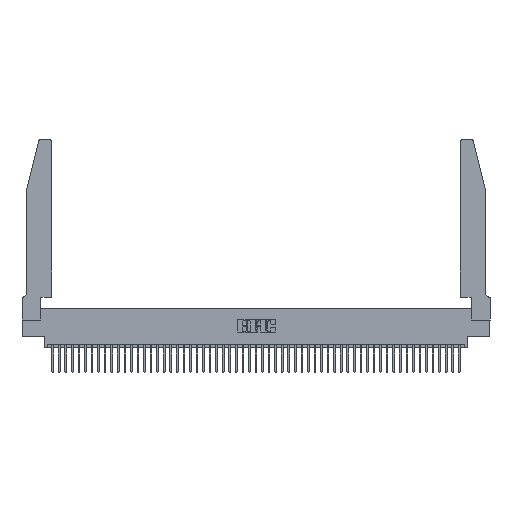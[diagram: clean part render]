
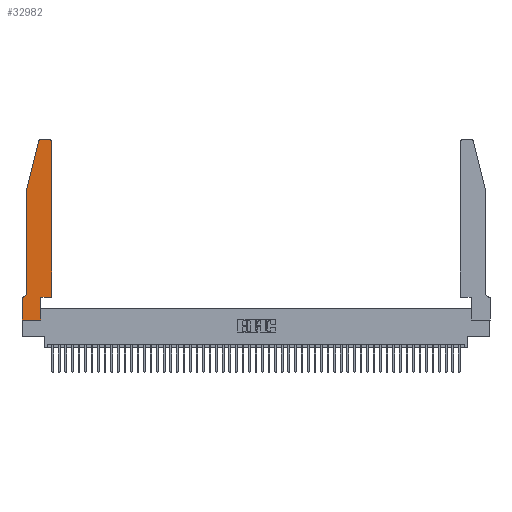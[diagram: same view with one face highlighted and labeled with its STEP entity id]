
A CAD part, top view. The second image highlights one B-rep face of the part: STEP entity #32982.
In plain terms, the highlighted planar face has unit normal (0, 0, 1).
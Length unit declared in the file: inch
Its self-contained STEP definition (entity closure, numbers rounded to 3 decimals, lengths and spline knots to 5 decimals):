
#950 = VERTEX_POINT ( 'NONE', #9124 ) ;
#957 = AXIS2_PLACEMENT_3D ( 'NONE', #36689, #12206, #44151 ) ;
#1061 = CARTESIAN_POINT ( 'NONE',  ( 0.0755, 2., 0.37 ) ) ;
#2277 = LINE ( 'NONE', #39306, #4116 ) ;
#3837 = AXIS2_PLACEMENT_3D ( 'NONE', #20028, #23515, #51494 ) ;
#4067 = ORIENTED_EDGE ( 'NONE', *, *, #48064, .T. ) ;
#4116 = VECTOR ( 'NONE', #31664, 39.37008 ) ;
#4285 = DIRECTION ( 'NONE',  ( 0., 1., 0. ) ) ;
#4808 = CIRCLE ( 'NONE', #3837, 0.03 ) ;
#4816 = DIRECTION ( 'NONE',  ( -1., 0., 0. ) ) ;
#5601 = VERTEX_POINT ( 'NONE', #50166 ) ;
#6028 = LINE ( 'NONE', #1061, #19692 ) ;
#6052 = LINE ( 'NONE', #10722, #41544 ) ;
#6655 = CARTESIAN_POINT ( 'NONE',  ( 0., 0., 0.37 ) ) ;
#6944 = EDGE_CURVE ( 'NONE', #26549, #43588, #12498, .T. ) ;
#7277 = ORIENTED_EDGE ( 'NONE', *, *, #22401, .T. ) ;
#8229 = VERTEX_POINT ( 'NONE', #43483 ) ;
#8336 = EDGE_CURVE ( 'NONE', #22446, #38537, #2277, .T. ) ;
#9124 = CARTESIAN_POINT ( 'NONE',  ( 0.4505, 0.35, 0.37 ) ) ;
#9871 = EDGE_CURVE ( 'NONE', #44445, #32906, #28897, .T. ) ;
#10722 = CARTESIAN_POINT ( 'NONE',  ( 0.2865, 0.35, 0.37 ) ) ;
#11219 = ORIENTED_EDGE ( 'NONE', *, *, #21768, .T. ) ;
#11962 = ORIENTED_EDGE ( 'NONE', *, *, #16718, .T. ) ;
#12115 = ORIENTED_EDGE ( 'NONE', *, *, #16935, .T. ) ;
#12206 = DIRECTION ( 'NONE',  ( 0., 0., -1. ) ) ;
#12373 = ORIENTED_EDGE ( 'NONE', *, *, #6944, .T. ) ;
#12456 = DIRECTION ( 'NONE',  ( 1., 0., 0. ) ) ;
#12498 = CIRCLE ( 'NONE', #21992, 0.03 ) ;
#12535 = VECTOR ( 'NONE', #22947, 39.37008 ) ;
#13772 = CARTESIAN_POINT ( 'NONE',  ( 0.4205, 2.75, 0.37 ) ) ;
#14092 = ORIENTED_EDGE ( 'NONE', *, *, #15169, .T. ) ;
#15169 = EDGE_CURVE ( 'NONE', #43588, #8229, #15907, .T. ) ;
#15867 = VERTEX_POINT ( 'NONE', #24768 ) ;
#15907 = LINE ( 'NONE', #48835, #21470 ) ;
#16263 = AXIS2_PLACEMENT_3D ( 'NONE', #42574, #50730, #50391 ) ;
#16718 = EDGE_CURVE ( 'NONE', #32906, #23641, #46926, .T. ) ;
#16935 = EDGE_CURVE ( 'NONE', #38537, #44445, #33230, .T. ) ;
#19171 = DIRECTION ( 'NONE',  ( 0., 1., 0. ) ) ;
#19416 = LINE ( 'NONE', #24122, #36853 ) ;
#19692 = VECTOR ( 'NONE', #33101, 39.37008 ) ;
#20028 = CARTESIAN_POINT ( 'NONE',  ( 0.284, 2.72, 0.37 ) ) ;
#21470 = VECTOR ( 'NONE', #4816, 39.37008 ) ;
#21768 = EDGE_CURVE ( 'NONE', #950, #26549, #19416, .T. ) ;
#21992 = AXIS2_PLACEMENT_3D ( 'NONE', #35269, #43443, #24112 ) ;
#22401 = EDGE_CURVE ( 'NONE', #51070, #950, #24958, .T. ) ;
#22446 = VERTEX_POINT ( 'NONE', #28395 ) ;
#22947 = DIRECTION ( 'NONE',  ( 1., 0., 0. ) ) ;
#23306 = ORIENTED_EDGE ( 'NONE', *, *, #45160, .T. ) ;
#23436 = EDGE_CURVE ( 'NONE', #23641, #15867, #34265, .T. ) ;
#23515 = DIRECTION ( 'NONE',  ( 0., 0., 1. ) ) ;
#23641 = VERTEX_POINT ( 'NONE', #32143 ) ;
#24112 = DIRECTION ( 'NONE',  ( 1., 0., 0. ) ) ;
#24122 = CARTESIAN_POINT ( 'NONE',  ( 0.4505, 0.35, 0.37 ) ) ;
#24768 = CARTESIAN_POINT ( 'NONE',  ( 0.2865, 0., 0.37 ) ) ;
#24958 = LINE ( 'NONE', #28742, #34312 ) ;
#25677 = CARTESIAN_POINT ( 'NONE',  ( 0.2865, 0.35, 0.37 ) ) ;
#26549 = VERTEX_POINT ( 'NONE', #33827 ) ;
#26898 = CARTESIAN_POINT ( 'NONE',  ( 0.0755, 0.35, 0.37 ) ) ;
#28395 = CARTESIAN_POINT ( 'NONE',  ( 0.0755, 2., 0.37 ) ) ;
#28742 = CARTESIAN_POINT ( 'NONE',  ( 0.4505, 0.35, 0.37 ) ) ;
#28818 = CARTESIAN_POINT ( 'NONE',  ( 0.0755, 0.42, 0.37 ) ) ;
#28897 = LINE ( 'NONE', #26898, #34498 ) ;
#30754 = PLANE ( 'NONE',  #16263 ) ;
#31664 = DIRECTION ( 'NONE',  ( 0., -1., 0. ) ) ;
#32143 = CARTESIAN_POINT ( 'NONE',  ( 0., 0., 0.37 ) ) ;
#32588 = ORIENTED_EDGE ( 'NONE', *, *, #8336, .T. ) ;
#32822 = FACE_OUTER_BOUND ( 'NONE', #48613, .T. ) ;
#32906 = VERTEX_POINT ( 'NONE', #33399 ) ;
#32982 = ADVANCED_FACE ( 'NONE', ( #32822 ), #30754, .T. ) ;
#33101 = DIRECTION ( 'NONE',  ( -0.239, -0.971, 0. ) ) ;
#33230 = CIRCLE ( 'NONE', #957, 0.07 ) ;
#33399 = CARTESIAN_POINT ( 'NONE',  ( 0., 0.35, 0.37 ) ) ;
#33827 = CARTESIAN_POINT ( 'NONE',  ( 0.4505, 2.72, 0.37 ) ) ;
#33848 = ORIENTED_EDGE ( 'NONE', *, *, #34353, .T. ) ;
#33868 = VECTOR ( 'NONE', #35148, 39.37008 ) ;
#34265 = LINE ( 'NONE', #50589, #12535 ) ;
#34312 = VECTOR ( 'NONE', #12456, 39.37008 ) ;
#34353 = EDGE_CURVE ( 'NONE', #5601, #22446, #6028, .T. ) ;
#34498 = VECTOR ( 'NONE', #50902, 39.37008 ) ;
#35148 = DIRECTION ( 'NONE',  ( 0., -1., 0. ) ) ;
#35269 = CARTESIAN_POINT ( 'NONE',  ( 0.4205, 2.72, 0.37 ) ) ;
#36689 = CARTESIAN_POINT ( 'NONE',  ( 0.0055, 0.42, 0.37 ) ) ;
#36853 = VECTOR ( 'NONE', #4285, 39.37008 ) ;
#38537 = VERTEX_POINT ( 'NONE', #28818 ) ;
#39306 = CARTESIAN_POINT ( 'NONE',  ( 0.0755, 2., 0.37 ) ) ;
#41544 = VECTOR ( 'NONE', #19171, 39.37008 ) ;
#41559 = ORIENTED_EDGE ( 'NONE', *, *, #23436, .T. ) ;
#42574 = CARTESIAN_POINT ( 'NONE',  ( 0., 0.35, 0.37 ) ) ;
#42706 = CARTESIAN_POINT ( 'NONE',  ( 0.0055, 0.35, 0.37 ) ) ;
#43443 = DIRECTION ( 'NONE',  ( 0., 0., 1. ) ) ;
#43483 = CARTESIAN_POINT ( 'NONE',  ( 0.284, 2.75, 0.37 ) ) ;
#43588 = VERTEX_POINT ( 'NONE', #13772 ) ;
#44151 = DIRECTION ( 'NONE',  ( -1., 0., 0. ) ) ;
#44445 = VERTEX_POINT ( 'NONE', #42706 ) ;
#45160 = EDGE_CURVE ( 'NONE', #8229, #5601, #4808, .T. ) ;
#46926 = LINE ( 'NONE', #6655, #33868 ) ;
#48064 = EDGE_CURVE ( 'NONE', #15867, #51070, #6052, .T. ) ;
#48613 = EDGE_LOOP ( 'NONE', ( #14092, #23306, #33848, #32588, #12115, #49544, #11962, #41559, #4067, #7277, #11219, #12373 ) ) ;
#48835 = CARTESIAN_POINT ( 'NONE',  ( 0.2605, 2.75, 0.37 ) ) ;
#49544 = ORIENTED_EDGE ( 'NONE', *, *, #9871, .T. ) ;
#50166 = CARTESIAN_POINT ( 'NONE',  ( 0.25487, 2.72718, 0.37 ) ) ;
#50391 = DIRECTION ( 'NONE',  ( 1., 0., 0. ) ) ;
#50589 = CARTESIAN_POINT ( 'NONE',  ( 0., 0., 0.37 ) ) ;
#50730 = DIRECTION ( 'NONE',  ( 0., 0., 1. ) ) ;
#50902 = DIRECTION ( 'NONE',  ( -1., 0., 0. ) ) ;
#51070 = VERTEX_POINT ( 'NONE', #25677 ) ;
#51494 = DIRECTION ( 'NONE',  ( 1., 0., 0. ) ) ;
